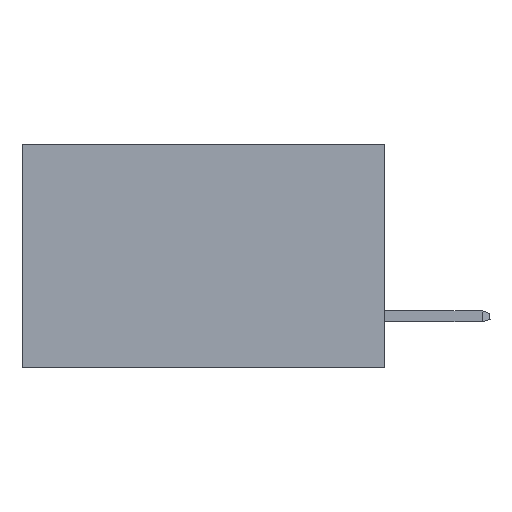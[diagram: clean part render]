
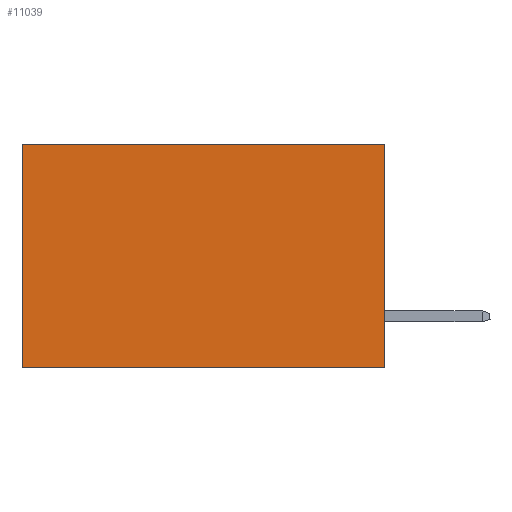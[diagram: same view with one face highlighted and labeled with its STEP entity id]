
A CAD part, left-side view. The second image highlights one B-rep face of the part: STEP entity #11039.
In plain terms, the highlighted planar face has unit normal (-1, 0, 0).
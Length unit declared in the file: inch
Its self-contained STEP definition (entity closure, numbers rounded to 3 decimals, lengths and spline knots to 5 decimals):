
#295 = CARTESIAN_POINT ( 'NONE',  ( 0.298, 0., 0. ) ) ;
#334 = EDGE_CURVE ( 'NONE', #3672, #5373, #10141, .T. ) ;
#908 = VERTEX_POINT ( 'NONE', #8493 ) ;
#1265 = DIRECTION ( 'NONE',  ( 0., 1., 0. ) ) ;
#2034 = EDGE_CURVE ( 'NONE', #12494, #908, #5360, .T. ) ;
#3535 = CARTESIAN_POINT ( 'NONE',  ( 0.298, 0., 0. ) ) ;
#3672 = VERTEX_POINT ( 'NONE', #4838 ) ;
#4659 = VECTOR ( 'NONE', #15994, 39.37008 ) ;
#4838 = CARTESIAN_POINT ( 'NONE',  ( 0.298, 0.6, 0. ) ) ;
#5360 = LINE ( 'NONE', #16510, #4659 ) ;
#5373 = VERTEX_POINT ( 'NONE', #12733 ) ;
#5446 = DIRECTION ( 'NONE',  ( 0., 0., -1. ) ) ;
#7350 = PLANE ( 'NONE',  #22026 ) ;
#8493 = CARTESIAN_POINT ( 'NONE',  ( 0.298, 0., -0.37 ) ) ;
#9277 = LINE ( 'NONE', #3535, #13958 ) ;
#9646 = DIRECTION ( 'NONE',  ( 1., 0., 0. ) ) ;
#10141 = LINE ( 'NONE', #17237, #28430 ) ;
#11039 = ADVANCED_FACE ( 'NONE', ( #12705 ), #7350, .F. ) ;
#12494 = VERTEX_POINT ( 'NONE', #26145 ) ;
#12705 = FACE_OUTER_BOUND ( 'NONE', #22646, .T. ) ;
#12733 = CARTESIAN_POINT ( 'NONE',  ( 0.298, 0.6, -0.37 ) ) ;
#13958 = VECTOR ( 'NONE', #21868, 39.37008 ) ;
#15313 = ORIENTED_EDGE ( 'NONE', *, *, #2034, .F. ) ;
#15666 = EDGE_CURVE ( 'NONE', #12494, #3672, #9277, .T. ) ;
#15994 = DIRECTION ( 'NONE',  ( 0., 0., -1. ) ) ;
#16510 = CARTESIAN_POINT ( 'NONE',  ( 0.298, 0., 0. ) ) ;
#17237 = CARTESIAN_POINT ( 'NONE',  ( 0.298, 0.6, 0. ) ) ;
#17303 = LINE ( 'NONE', #17428, #23387 ) ;
#17428 = CARTESIAN_POINT ( 'NONE',  ( 0.298, 0., -0.37 ) ) ;
#17718 = ORIENTED_EDGE ( 'NONE', *, *, #24595, .F. ) ;
#21868 = DIRECTION ( 'NONE',  ( 0., 1., 0. ) ) ;
#22026 = AXIS2_PLACEMENT_3D ( 'NONE', #295, #9646, #25712 ) ;
#22646 = EDGE_LOOP ( 'NONE', ( #24335, #17718, #15313, #23715 ) ) ;
#23387 = VECTOR ( 'NONE', #1265, 39.37008 ) ;
#23715 = ORIENTED_EDGE ( 'NONE', *, *, #15666, .T. ) ;
#24335 = ORIENTED_EDGE ( 'NONE', *, *, #334, .T. ) ;
#24595 = EDGE_CURVE ( 'NONE', #908, #5373, #17303, .T. ) ;
#25712 = DIRECTION ( 'NONE',  ( 0., 0., -1. ) ) ;
#26145 = CARTESIAN_POINT ( 'NONE',  ( 0.298, 0., 0. ) ) ;
#28430 = VECTOR ( 'NONE', #5446, 39.37008 ) ;
